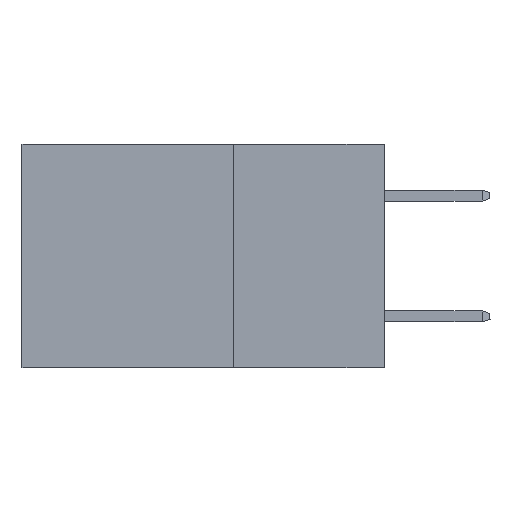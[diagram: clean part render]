
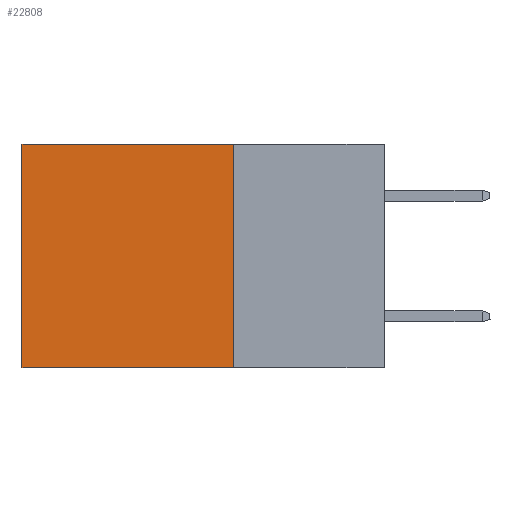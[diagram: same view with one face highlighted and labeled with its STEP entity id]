
A CAD part, left-side view. The second image highlights one B-rep face of the part: STEP entity #22808.
In plain terms, the highlighted planar face has unit normal (-1, 0, 0).
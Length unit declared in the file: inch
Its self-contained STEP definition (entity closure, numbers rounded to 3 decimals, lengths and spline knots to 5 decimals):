
#285 = LINE ( 'NONE', #23008, #20833 ) ;
#425 = DIRECTION ( 'NONE',  ( 1., 0., 0. ) ) ;
#778 = DIRECTION ( 'NONE',  ( 0., 1., 0. ) ) ;
#1716 = CARTESIAN_POINT ( 'NONE',  ( 0.2615, 0.6, -0.37 ) ) ;
#3167 = ORIENTED_EDGE ( 'NONE', *, *, #11079, .F. ) ;
#3201 = DIRECTION ( 'NONE',  ( 0., 0., -1. ) ) ;
#5806 = EDGE_LOOP ( 'NONE', ( #13493, #3167, #15877, #16077 ) ) ;
#6842 = VERTEX_POINT ( 'NONE', #1716 ) ;
#7551 = LINE ( 'NONE', #10901, #22628 ) ;
#7921 = EDGE_CURVE ( 'NONE', #13543, #9205, #7551, .T. ) ;
#8809 = CARTESIAN_POINT ( 'NONE',  ( 0.2615, 0.25, 0. ) ) ;
#9205 = VERTEX_POINT ( 'NONE', #10851 ) ;
#10273 = FACE_OUTER_BOUND ( 'NONE', #5806, .T. ) ;
#10851 = CARTESIAN_POINT ( 'NONE',  ( 0.2615, 0.6, 0. ) ) ;
#10901 = CARTESIAN_POINT ( 'NONE',  ( 0.2615, 0.25, 0. ) ) ;
#11079 = EDGE_CURVE ( 'NONE', #17608, #6842, #24584, .T. ) ;
#12563 = CARTESIAN_POINT ( 'NONE',  ( 0.2615, 0.25, -0.37 ) ) ;
#13235 = CARTESIAN_POINT ( 'NONE',  ( 0.2615, 0.25, -0.37 ) ) ;
#13493 = ORIENTED_EDGE ( 'NONE', *, *, #17199, .T. ) ;
#13543 = VERTEX_POINT ( 'NONE', #8809 ) ;
#13544 = AXIS2_PLACEMENT_3D ( 'NONE', #12563, #425, #14520 ) ;
#14451 = CARTESIAN_POINT ( 'NONE',  ( 0.2615, 0.25, -0.37 ) ) ;
#14520 = DIRECTION ( 'NONE',  ( 0., 0., -1. ) ) ;
#15877 = ORIENTED_EDGE ( 'NONE', *, *, #20123, .F. ) ;
#16077 = ORIENTED_EDGE ( 'NONE', *, *, #7921, .T. ) ;
#16536 = LINE ( 'NONE', #13235, #21053 ) ;
#17199 = EDGE_CURVE ( 'NONE', #9205, #6842, #285, .T. ) ;
#17608 = VERTEX_POINT ( 'NONE', #14451 ) ;
#17643 = DIRECTION ( 'NONE',  ( 0., 1., 0. ) ) ;
#19470 = VECTOR ( 'NONE', #17643, 39.37008 ) ;
#20123 = EDGE_CURVE ( 'NONE', #13543, #17608, #16536, .T. ) ;
#20833 = VECTOR ( 'NONE', #24908, 39.37008 ) ;
#21053 = VECTOR ( 'NONE', #3201, 39.37008 ) ;
#22628 = VECTOR ( 'NONE', #778, 39.37008 ) ;
#22808 = ADVANCED_FACE ( 'NONE', ( #10273 ), #24144, .F. ) ;
#23008 = CARTESIAN_POINT ( 'NONE',  ( 0.2615, 0.6, -0.37 ) ) ;
#24144 = PLANE ( 'NONE',  #13544 ) ;
#24584 = LINE ( 'NONE', #25275, #19470 ) ;
#24908 = DIRECTION ( 'NONE',  ( 0., 0., -1. ) ) ;
#25275 = CARTESIAN_POINT ( 'NONE',  ( 0.2615, 0.25, -0.37 ) ) ;
